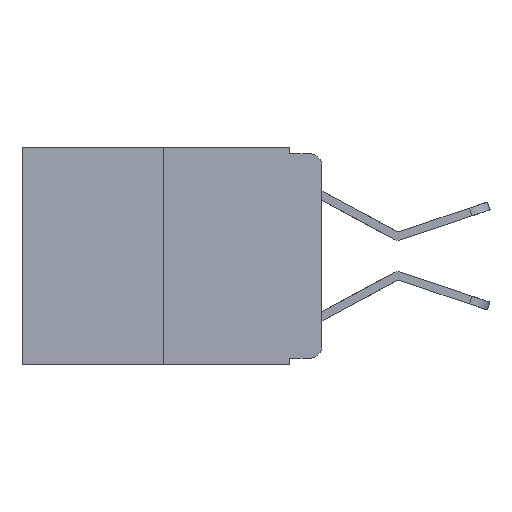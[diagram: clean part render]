
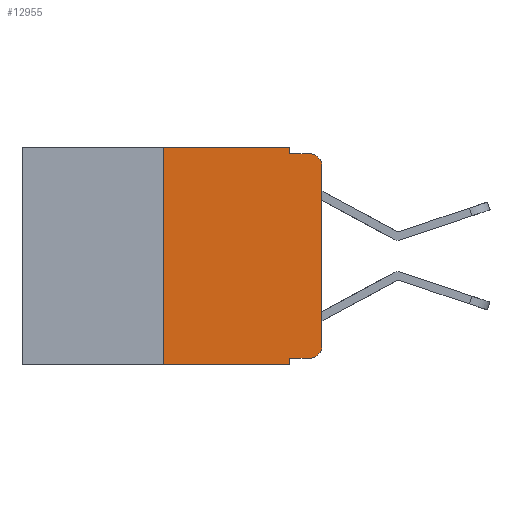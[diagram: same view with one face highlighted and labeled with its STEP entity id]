
A CAD part, left-side view. The second image highlights one B-rep face of the part: STEP entity #12955.
In plain terms, the highlighted planar face has unit normal (-1, 0, 0).
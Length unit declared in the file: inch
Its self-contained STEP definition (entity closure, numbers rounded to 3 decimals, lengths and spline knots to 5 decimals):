
#265 = DIRECTION ( 'NONE',  ( 0., -1., 0. ) ) ;
#301 = EDGE_CURVE ( 'NONE', #3347, #10080, #1549, .T. ) ;
#410 = AXIS2_PLACEMENT_3D ( 'NONE', #3532, #6766, #14133 ) ;
#755 = VERTEX_POINT ( 'NONE', #6829 ) ;
#1146 = EDGE_CURVE ( 'NONE', #755, #10080, #7997, .T. ) ;
#1164 = EDGE_LOOP ( 'NONE', ( #14070, #12301, #1347, #8005, #5475, #11473, #11800, #9372, #4299, #5653 ) ) ;
#1347 = ORIENTED_EDGE ( 'NONE', *, *, #301, .F. ) ;
#1422 = VERTEX_POINT ( 'NONE', #11597 ) ;
#1549 = LINE ( 'NONE', #11738, #10339 ) ;
#1985 = EDGE_CURVE ( 'NONE', #11092, #755, #5245, .T. ) ;
#1997 = CARTESIAN_POINT ( 'NONE',  ( 0., 0.051, -0.01 ) ) ;
#2309 = DIRECTION ( 'NONE',  ( -1., 0., 0. ) ) ;
#2334 = CARTESIAN_POINT ( 'NONE',  ( 0., 0.25, 0. ) ) ;
#2414 = VERTEX_POINT ( 'NONE', #8974 ) ;
#2854 = CARTESIAN_POINT ( 'NONE',  ( 0., 0.25, 0. ) ) ;
#3347 = VERTEX_POINT ( 'NONE', #1997 ) ;
#3460 = DIRECTION ( 'NONE',  ( 0., 0., -1. ) ) ;
#3532 = CARTESIAN_POINT ( 'NONE',  ( 0., 0.473, 0. ) ) ;
#3534 = VERTEX_POINT ( 'NONE', #2334 ) ;
#3586 = LINE ( 'NONE', #10434, #6089 ) ;
#4099 = FACE_OUTER_BOUND ( 'NONE', #1164, .T. ) ;
#4244 = CARTESIAN_POINT ( 'NONE',  ( 0., 0.473, 0. ) ) ;
#4299 = ORIENTED_EDGE ( 'NONE', *, *, #11719, .T. ) ;
#4406 = LINE ( 'NONE', #5020, #7267 ) ;
#4821 = CARTESIAN_POINT ( 'NONE',  ( 0., 0., 0. ) ) ;
#4973 = DIRECTION ( 'NONE',  ( -1., 0., 0. ) ) ;
#5020 = CARTESIAN_POINT ( 'NONE',  ( 0., 0.473, -0.343 ) ) ;
#5084 = DIRECTION ( 'NONE',  ( 0., 0., -1. ) ) ;
#5245 = LINE ( 'NONE', #4821, #10605 ) ;
#5475 = ORIENTED_EDGE ( 'NONE', *, *, #9303, .F. ) ;
#5653 = ORIENTED_EDGE ( 'NONE', *, *, #10312, .T. ) ;
#5711 = VECTOR ( 'NONE', #12760, 39.37008 ) ;
#5812 = LINE ( 'NONE', #7106, #11154 ) ;
#6089 = VECTOR ( 'NONE', #5084, 39.37008 ) ;
#6198 = EDGE_CURVE ( 'NONE', #6474, #9232, #4406, .T. ) ;
#6352 = CIRCLE ( 'NONE', #13469, 0.02 ) ;
#6468 = CARTESIAN_POINT ( 'NONE',  ( 0., 0.25, -0.343 ) ) ;
#6474 = VERTEX_POINT ( 'NONE', #6468 ) ;
#6766 = DIRECTION ( 'NONE',  ( 1., 0., 0. ) ) ;
#6829 = CARTESIAN_POINT ( 'NONE',  ( 0., 0., -0.03 ) ) ;
#7106 = CARTESIAN_POINT ( 'NONE',  ( 0., 0.051, -0.333 ) ) ;
#7267 = VECTOR ( 'NONE', #11409, 39.37008 ) ;
#7997 = CIRCLE ( 'NONE', #13875, 0.02 ) ;
#8005 = ORIENTED_EDGE ( 'NONE', *, *, #13808, .F. ) ;
#8451 = CARTESIAN_POINT ( 'NONE',  ( 0., 0.051, -0.343 ) ) ;
#8751 = CARTESIAN_POINT ( 'NONE',  ( 0., 0.02, -0.333 ) ) ;
#8928 = CARTESIAN_POINT ( 'NONE',  ( 0., 0.02, -0.03 ) ) ;
#8974 = CARTESIAN_POINT ( 'NONE',  ( 0., 0.051, 0. ) ) ;
#9232 = VERTEX_POINT ( 'NONE', #8451 ) ;
#9303 = EDGE_CURVE ( 'NONE', #3534, #2414, #11701, .T. ) ;
#9322 = DIRECTION ( 'NONE',  ( 0., 0., 1. ) ) ;
#9355 = CARTESIAN_POINT ( 'NONE',  ( 0., 0., -0.313 ) ) ;
#9372 = ORIENTED_EDGE ( 'NONE', *, *, #12429, .F. ) ;
#9513 = LINE ( 'NONE', #11285, #11947 ) ;
#10080 = VERTEX_POINT ( 'NONE', #10976 ) ;
#10312 = EDGE_CURVE ( 'NONE', #12858, #11092, #6352, .T. ) ;
#10339 = VECTOR ( 'NONE', #13253, 39.37008 ) ;
#10434 = CARTESIAN_POINT ( 'NONE',  ( 0., 0.051, 0. ) ) ;
#10605 = VECTOR ( 'NONE', #11235, 39.37008 ) ;
#10619 = VECTOR ( 'NONE', #9322, 39.37008 ) ;
#10965 = LINE ( 'NONE', #2854, #10619 ) ;
#10976 = CARTESIAN_POINT ( 'NONE',  ( 0., 0.02, -0.01 ) ) ;
#11092 = VERTEX_POINT ( 'NONE', #9355 ) ;
#11154 = VECTOR ( 'NONE', #265, 39.37008 ) ;
#11235 = DIRECTION ( 'NONE',  ( 0., 0., 1. ) ) ;
#11285 = CARTESIAN_POINT ( 'NONE',  ( 0., 0.051, 0. ) ) ;
#11375 = CARTESIAN_POINT ( 'NONE',  ( 0., 0.02, -0.313 ) ) ;
#11409 = DIRECTION ( 'NONE',  ( 0., -1., 0. ) ) ;
#11473 = ORIENTED_EDGE ( 'NONE', *, *, #13136, .F. ) ;
#11597 = CARTESIAN_POINT ( 'NONE',  ( 0., 0.051, -0.333 ) ) ;
#11701 = LINE ( 'NONE', #4244, #5711 ) ;
#11719 = EDGE_CURVE ( 'NONE', #1422, #12858, #5812, .T. ) ;
#11738 = CARTESIAN_POINT ( 'NONE',  ( 0., 0.051, -0.01 ) ) ;
#11800 = ORIENTED_EDGE ( 'NONE', *, *, #6198, .T. ) ;
#11947 = VECTOR ( 'NONE', #12394, 39.37008 ) ;
#12301 = ORIENTED_EDGE ( 'NONE', *, *, #1146, .T. ) ;
#12394 = DIRECTION ( 'NONE',  ( 0., 0., -1. ) ) ;
#12429 = EDGE_CURVE ( 'NONE', #1422, #9232, #9513, .T. ) ;
#12432 = DIRECTION ( 'NONE',  ( 0., 0., -1. ) ) ;
#12760 = DIRECTION ( 'NONE',  ( 0., -1., 0. ) ) ;
#12858 = VERTEX_POINT ( 'NONE', #8751 ) ;
#12955 = ADVANCED_FACE ( 'NONE', ( #4099 ), #13112, .F. ) ;
#13112 = PLANE ( 'NONE',  #410 ) ;
#13136 = EDGE_CURVE ( 'NONE', #6474, #3534, #10965, .T. ) ;
#13253 = DIRECTION ( 'NONE',  ( 0., -1., 0. ) ) ;
#13469 = AXIS2_PLACEMENT_3D ( 'NONE', #11375, #4973, #12432 ) ;
#13808 = EDGE_CURVE ( 'NONE', #2414, #3347, #3586, .T. ) ;
#13875 = AXIS2_PLACEMENT_3D ( 'NONE', #8928, #2309, #3460 ) ;
#14070 = ORIENTED_EDGE ( 'NONE', *, *, #1985, .T. ) ;
#14133 = DIRECTION ( 'NONE',  ( 0., 0., -1. ) ) ;
